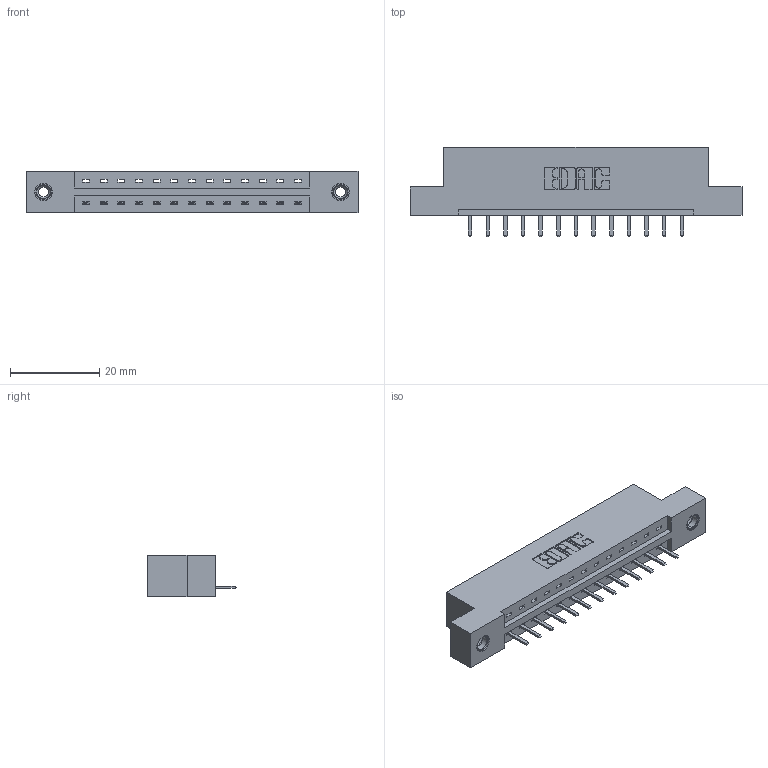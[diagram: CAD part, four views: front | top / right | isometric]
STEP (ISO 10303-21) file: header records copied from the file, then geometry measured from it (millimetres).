
FILE_DESCRIPTION (( 'STEP AP203' ), '1' );
FILE_NAME ('387-013-520-108.STEP', '2019-10-02T13:50:44', ( '' ), ( '' ), 'SwSTEP 2.0', 'SolidWorks 2016', '' );
FILE_SCHEMA (( 'CONFIG_CONTROL_DESIGN' ));
Length unit declared in the file: inch
Products named in the file (4): 387-013-520-108; 337 Part_Flush Mounting Lugs - 0.156 Dia-TI; 345-292-001_345-293-120; 345-250-001_345-250-003-102
Assembly tree (16 placements, depth 2):
  387-013-520-108
    337 Part_Flush Mounting Lugs - 0.156 Dia-TI
    345-292-001_345-293-120  x13
    345-250-001_345-250-003-102  x2
Bounding box: 74.52 x 20.02 x 9.4 mm (x, y, z)
Volume: 7338.7 mm3; surface area: 7317.6 mm2
Topology: 16 solids, 16 shells, 1032 faces, 2995 edges, 1954 vertices
Faces by surface type: plane 726, cylinder 290, cone 12, torus 4
Entity records: 14714 total; most frequent: CARTESIAN_POINT 2552, ORIENTED_EDGE 2482, DIRECTION 2229, EDGE_CURVE 1241, VECTOR 1089, LINE 1089, VERTEX_POINT 820, AXIS2_PLACEMENT_3D 570
